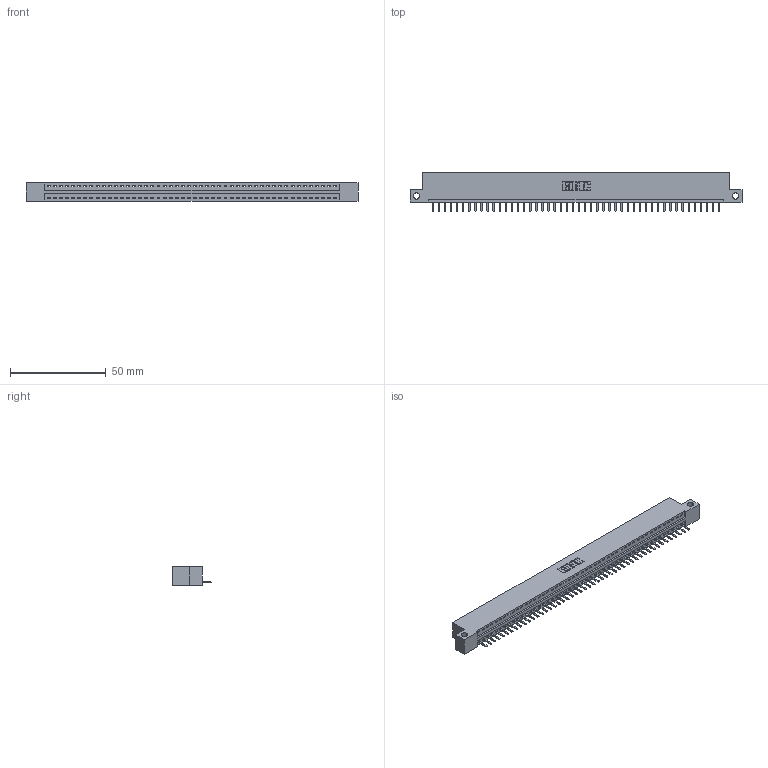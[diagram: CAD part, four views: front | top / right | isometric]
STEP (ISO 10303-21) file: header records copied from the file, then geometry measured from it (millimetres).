
FILE_DESCRIPTION (( 'STEP AP203' ), '1' );
FILE_NAME ('346-048-520-112.STEP', '2022-05-09T22:56:28', ( '' ), ( '' ), 'SwSTEP 2.0', 'SolidWorks 2020', '' );
FILE_SCHEMA (( 'CONFIG_CONTROL_DESIGN' ));
Length unit declared in the file: inch
Products named in the file (3): 346 Part_Flush Mounting Lugs - Side Mount; 345-292-001_345-293-120; 346-048-520-112
Assembly tree (49 placements, depth 2):
  346-048-520-112
    346 Part_Flush Mounting Lugs - Side Mount
    345-292-001_345-293-120  x48
Bounding box: 172.97 x 20.02 x 9.4 mm (x, y, z)
Volume: 410.8 mm3; surface area: 19850.5 mm2
Topology: 48 solids, 49 shells, 3092 faces, 9160 edges, 5978 vertices
Faces by surface type: plane 2086, cylinder 1006
Entity records: 29099 total; most frequent: CARTESIAN_POINT 5004, ORIENTED_EDGE 4974, DIRECTION 4395, EDGE_CURVE 2487, VECTOR 2159, LINE 2159, VERTEX_POINT 1654, AXIS2_PLACEMENT_3D 1118
